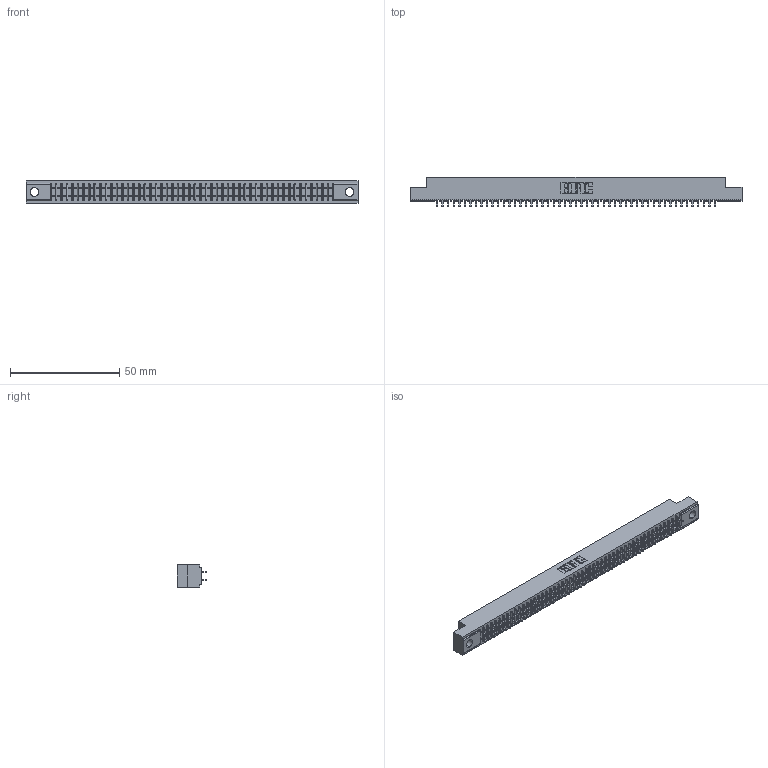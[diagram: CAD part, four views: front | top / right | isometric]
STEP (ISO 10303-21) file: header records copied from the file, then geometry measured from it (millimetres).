
FILE_DESCRIPTION (( 'STEP AP203' ), '1' );
FILE_NAME ('341-102-524-204.STEP', '2018-08-08T11:13:43', ( '' ), ( '' ), 'SwSTEP 2.0', 'SolidWorks 2016', '' );
FILE_SCHEMA (( 'CONFIG_CONTROL_DESIGN' ));
Length unit declared in the file: inch
Products named in the file (3): 341 Part_.156 (3.96) Dia Mounting Holes; 341-292-001_341-292-124; 341-102-524-204
Assembly tree (103 placements, depth 2):
  341-102-524-204
    341 Part_.156 (3.96) Dia Mounting Holes
    341-292-001_341-292-124  x102
Bounding box: 151.76 x 13.64 x 10.16 mm (x, y, z)
Volume: 11099.5 mm3; surface area: 19676.8 mm2
Topology: 103 solids, 103 shells, 6862 faces, 19885 edges, 12878 vertices
Faces by surface type: plane 4162, cylinder 2496, sphere 104, torus 100
Entity records: 60940 total; most frequent: CARTESIAN_POINT 10135, ORIENTED_EDGE 10070, DIRECTION 9821, EDGE_CURVE 5035, VECTOR 4085, LINE 4085, VERTEX_POINT 3182, AXIS2_PLACEMENT_3D 2868
